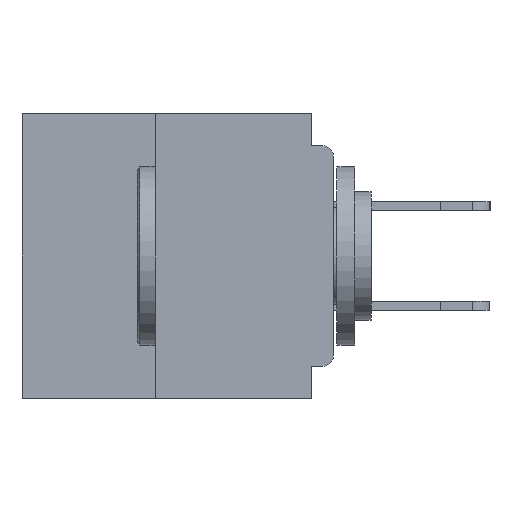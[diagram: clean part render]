
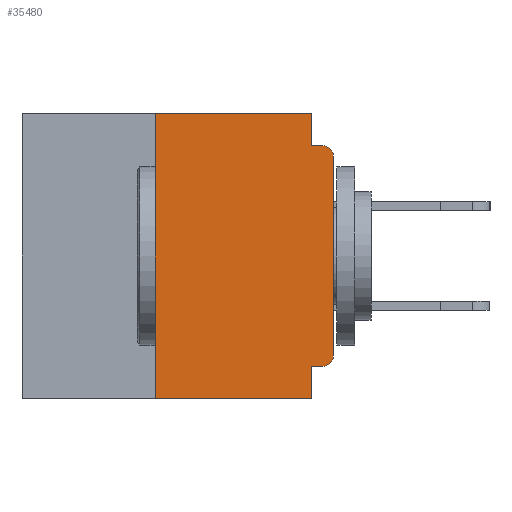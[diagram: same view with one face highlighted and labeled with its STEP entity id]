
A CAD part, left-side view. The second image highlights one B-rep face of the part: STEP entity #35480.
In plain terms, the highlighted planar face has unit normal (-1, 0, 0).
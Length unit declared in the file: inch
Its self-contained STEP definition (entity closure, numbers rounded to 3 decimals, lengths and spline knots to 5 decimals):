
#150 = AXIS2_PLACEMENT_3D ( 'NONE', #23295, #41772, #14260 ) ;
#2149 = DIRECTION ( 'NONE',  ( -1., 0., 0. ) ) ;
#2350 = AXIS2_PLACEMENT_3D ( 'NONE', #29644, #2149, #34283 ) ;
#3366 = EDGE_CURVE ( 'NONE', #37213, #26608, #52524, .T. ) ;
#3440 = EDGE_CURVE ( 'NONE', #22465, #27323, #38930, .T. ) ;
#3712 = VECTOR ( 'NONE', #22598, 39.37008 ) ;
#3715 = ORIENTED_EDGE ( 'NONE', *, *, #4949, .F. ) ;
#4949 = EDGE_CURVE ( 'NONE', #23210, #26608, #26594, .T. ) ;
#5167 = CARTESIAN_POINT ( 'NONE',  ( 0., 0.031, -0.045 ) ) ;
#6959 = FACE_OUTER_BOUND ( 'NONE', #54236, .T. ) ;
#8526 = ORIENTED_EDGE ( 'NONE', *, *, #24295, .T. ) ;
#9694 = CARTESIAN_POINT ( 'NONE',  ( 0., 0., -0.34 ) ) ;
#9943 = EDGE_CURVE ( 'NONE', #11742, #44467, #30350, .T. ) ;
#10502 = LINE ( 'NONE', #24425, #32088 ) ;
#11117 = VERTEX_POINT ( 'NONE', #43019 ) ;
#11742 = VERTEX_POINT ( 'NONE', #55719 ) ;
#12521 = CARTESIAN_POINT ( 'NONE',  ( 0., 0., -0.355 ) ) ;
#12865 = ORIENTED_EDGE ( 'NONE', *, *, #3440, .F. ) ;
#13049 = DIRECTION ( 'NONE',  ( 0., 1., 0. ) ) ;
#13173 = LINE ( 'NONE', #33457, #36152 ) ;
#13331 = CARTESIAN_POINT ( 'NONE',  ( 0., 0.25, -0.4 ) ) ;
#13750 = LINE ( 'NONE', #13331, #25992 ) ;
#13863 = DIRECTION ( 'NONE',  ( 0., 0., 1. ) ) ;
#14143 = DIRECTION ( 'NONE',  ( 0., 0., -1. ) ) ;
#14220 = DIRECTION ( 'NONE',  ( -1., 0., 0. ) ) ;
#14260 = DIRECTION ( 'NONE',  ( 0., 0., -1. ) ) ;
#14310 = CARTESIAN_POINT ( 'NONE',  ( 0., 0.015, -0.06 ) ) ;
#14482 = VECTOR ( 'NONE', #13049, 39.37008 ) ;
#14608 = ORIENTED_EDGE ( 'NONE', *, *, #3366, .T. ) ;
#17525 = ORIENTED_EDGE ( 'NONE', *, *, #32474, .T. ) ;
#19000 = CIRCLE ( 'NONE', #2350, 0.015 ) ;
#21272 = CARTESIAN_POINT ( 'NONE',  ( 0., 0.437, -0.4 ) ) ;
#22465 = VERTEX_POINT ( 'NONE', #46092 ) ;
#22598 = DIRECTION ( 'NONE',  ( 0., 0., -1. ) ) ;
#23210 = VERTEX_POINT ( 'NONE', #5167 ) ;
#23295 = CARTESIAN_POINT ( 'NONE',  ( 0., 0.437, 0. ) ) ;
#23812 = VERTEX_POINT ( 'NONE', #9694 ) ;
#24295 = EDGE_CURVE ( 'NONE', #23812, #37213, #41256, .T. ) ;
#24414 = DIRECTION ( 'NONE',  ( 0., 0., -1. ) ) ;
#24425 = CARTESIAN_POINT ( 'NONE',  ( 0., 0.437, 0. ) ) ;
#25187 = ORIENTED_EDGE ( 'NONE', *, *, #38262, .F. ) ;
#25902 = DIRECTION ( 'NONE',  ( 0., -1., 0. ) ) ;
#25992 = VECTOR ( 'NONE', #36407, 39.37008 ) ;
#26594 = LINE ( 'NONE', #31786, #48112 ) ;
#26608 = VERTEX_POINT ( 'NONE', #55566 ) ;
#27323 = VERTEX_POINT ( 'NONE', #51893 ) ;
#27725 = CARTESIAN_POINT ( 'NONE',  ( 0., 0., 0. ) ) ;
#27930 = PLANE ( 'NONE',  #150 ) ;
#29644 = CARTESIAN_POINT ( 'NONE',  ( 0., 0.015, -0.34 ) ) ;
#30350 = LINE ( 'NONE', #21272, #53296 ) ;
#30634 = ORIENTED_EDGE ( 'NONE', *, *, #55726, .F. ) ;
#31195 = DIRECTION ( 'NONE',  ( 0., -1., 0. ) ) ;
#31786 = CARTESIAN_POINT ( 'NONE',  ( 0., 0., -0.045 ) ) ;
#32073 = VERTEX_POINT ( 'NONE', #49376 ) ;
#32088 = VECTOR ( 'NONE', #47493, 39.37008 ) ;
#32474 = EDGE_CURVE ( 'NONE', #22465, #23812, #19000, .T. ) ;
#33457 = CARTESIAN_POINT ( 'NONE',  ( 0., 0.031, -0.4 ) ) ;
#34283 = DIRECTION ( 'NONE',  ( 0., 0., -1. ) ) ;
#34299 = ORIENTED_EDGE ( 'NONE', *, *, #45837, .F. ) ;
#35480 = ADVANCED_FACE ( 'NONE', ( #6959 ), #27930, .F. ) ;
#36152 = VECTOR ( 'NONE', #24414, 39.37008 ) ;
#36407 = DIRECTION ( 'NONE',  ( 0., 0., 1. ) ) ;
#37213 = VERTEX_POINT ( 'NONE', #44997 ) ;
#38262 = EDGE_CURVE ( 'NONE', #11742, #32073, #13750, .T. ) ;
#38897 = LINE ( 'NONE', #50089, #3712 ) ;
#38930 = LINE ( 'NONE', #12521, #14482 ) ;
#41110 = AXIS2_PLACEMENT_3D ( 'NONE', #14310, #14220, #14143 ) ;
#41256 = LINE ( 'NONE', #27725, #50549 ) ;
#41772 = DIRECTION ( 'NONE',  ( 1., 0., 0. ) ) ;
#42152 = EDGE_CURVE ( 'NONE', #32073, #11117, #10502, .T. ) ;
#43019 = CARTESIAN_POINT ( 'NONE',  ( 0., 0.031, 0. ) ) ;
#44467 = VERTEX_POINT ( 'NONE', #58430 ) ;
#44997 = CARTESIAN_POINT ( 'NONE',  ( 0., 0., -0.06 ) ) ;
#45543 = ORIENTED_EDGE ( 'NONE', *, *, #9943, .T. ) ;
#45837 = EDGE_CURVE ( 'NONE', #11117, #23210, #38897, .T. ) ;
#46092 = CARTESIAN_POINT ( 'NONE',  ( 0., 0.015, -0.355 ) ) ;
#46758 = ORIENTED_EDGE ( 'NONE', *, *, #42152, .F. ) ;
#47493 = DIRECTION ( 'NONE',  ( 0., -1., 0. ) ) ;
#48112 = VECTOR ( 'NONE', #31195, 39.37008 ) ;
#49376 = CARTESIAN_POINT ( 'NONE',  ( 0., 0.25, 0. ) ) ;
#50089 = CARTESIAN_POINT ( 'NONE',  ( 0., 0.031, 0. ) ) ;
#50549 = VECTOR ( 'NONE', #13863, 39.37008 ) ;
#51893 = CARTESIAN_POINT ( 'NONE',  ( 0., 0.031, -0.355 ) ) ;
#52524 = CIRCLE ( 'NONE', #41110, 0.015 ) ;
#53296 = VECTOR ( 'NONE', #25902, 39.37008 ) ;
#54236 = EDGE_LOOP ( 'NONE', ( #8526, #14608, #3715, #34299, #46758, #25187, #45543, #30634, #12865, #17525 ) ) ;
#55566 = CARTESIAN_POINT ( 'NONE',  ( 0., 0.015, -0.045 ) ) ;
#55719 = CARTESIAN_POINT ( 'NONE',  ( 0., 0.25, -0.4 ) ) ;
#55726 = EDGE_CURVE ( 'NONE', #27323, #44467, #13173, .T. ) ;
#58430 = CARTESIAN_POINT ( 'NONE',  ( 0., 0.031, -0.4 ) ) ;
